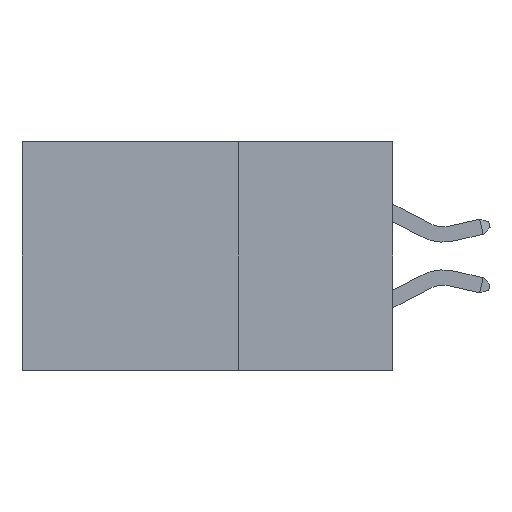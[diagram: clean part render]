
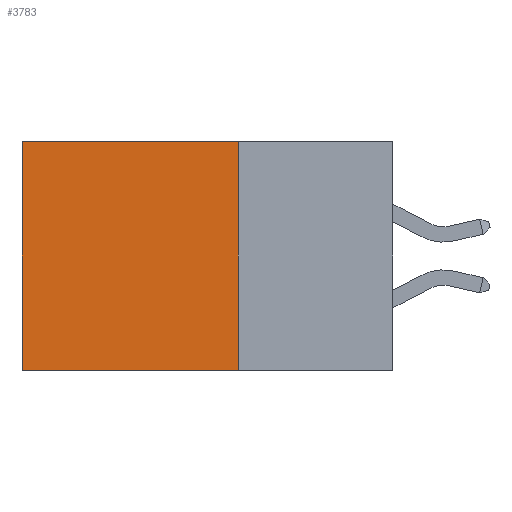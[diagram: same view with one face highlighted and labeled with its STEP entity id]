
A CAD part, left-side view. The second image highlights one B-rep face of the part: STEP entity #3783.
In plain terms, the highlighted planar face has unit normal (-1, 0, 0).
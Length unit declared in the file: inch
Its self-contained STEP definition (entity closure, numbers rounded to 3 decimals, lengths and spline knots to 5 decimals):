
#979 = ORIENTED_EDGE ( 'NONE', *, *, #10475, .F. ) ;
#1186 = DIRECTION ( 'NONE',  ( 0., 0., -1. ) ) ;
#1193 = VERTEX_POINT ( 'NONE', #20243 ) ;
#2127 = CARTESIAN_POINT ( 'NONE',  ( 0.2875, 0.6, -0.37 ) ) ;
#2405 = CARTESIAN_POINT ( 'NONE',  ( 0.2875, 0.25, -0.37 ) ) ;
#2890 = LINE ( 'NONE', #20522, #14597 ) ;
#3520 = VERTEX_POINT ( 'NONE', #20196 ) ;
#3783 = ADVANCED_FACE ( 'NONE', ( #15075 ), #10285, .F. ) ;
#3877 = VERTEX_POINT ( 'NONE', #4519 ) ;
#4420 = LINE ( 'NONE', #15878, #14667 ) ;
#4519 = CARTESIAN_POINT ( 'NONE',  ( 0.2875, 0.6, 0. ) ) ;
#4660 = DIRECTION ( 'NONE',  ( 0., 1., 0. ) ) ;
#7227 = DIRECTION ( 'NONE',  ( 1., 0., 0. ) ) ;
#8703 = DIRECTION ( 'NONE',  ( 0., 0., -1. ) ) ;
#9340 = ORIENTED_EDGE ( 'NONE', *, *, #15856, .T. ) ;
#9918 = VERTEX_POINT ( 'NONE', #2127 ) ;
#10285 = PLANE ( 'NONE',  #14788 ) ;
#10475 = EDGE_CURVE ( 'NONE', #1193, #9918, #16786, .T. ) ;
#11644 = EDGE_LOOP ( 'NONE', ( #9340, #979, #19516, #18137 ) ) ;
#11767 = VECTOR ( 'NONE', #12009, 39.37008 ) ;
#12009 = DIRECTION ( 'NONE',  ( 0., 1., 0. ) ) ;
#13523 = CARTESIAN_POINT ( 'NONE',  ( 0.2875, 0.6, 0. ) ) ;
#13703 = EDGE_CURVE ( 'NONE', #3520, #3877, #2890, .T. ) ;
#14597 = VECTOR ( 'NONE', #4660, 39.37008 ) ;
#14667 = VECTOR ( 'NONE', #1186, 39.37008 ) ;
#14788 = AXIS2_PLACEMENT_3D ( 'NONE', #16624, #7227, #8703 ) ;
#15075 = FACE_OUTER_BOUND ( 'NONE', #11644, .T. ) ;
#15856 = EDGE_CURVE ( 'NONE', #3877, #9918, #18198, .T. ) ;
#15878 = CARTESIAN_POINT ( 'NONE',  ( 0.2875, 0.25, 0. ) ) ;
#15972 = EDGE_CURVE ( 'NONE', #3520, #1193, #4420, .T. ) ;
#16624 = CARTESIAN_POINT ( 'NONE',  ( 0.2875, 0.25, 0. ) ) ;
#16786 = LINE ( 'NONE', #2405, #11767 ) ;
#18137 = ORIENTED_EDGE ( 'NONE', *, *, #13703, .T. ) ;
#18198 = LINE ( 'NONE', #13523, #18632 ) ;
#18632 = VECTOR ( 'NONE', #19864, 39.37008 ) ;
#19516 = ORIENTED_EDGE ( 'NONE', *, *, #15972, .F. ) ;
#19864 = DIRECTION ( 'NONE',  ( 0., 0., -1. ) ) ;
#20196 = CARTESIAN_POINT ( 'NONE',  ( 0.2875, 0.25, 0. ) ) ;
#20243 = CARTESIAN_POINT ( 'NONE',  ( 0.2875, 0.25, -0.37 ) ) ;
#20522 = CARTESIAN_POINT ( 'NONE',  ( 0.2875, 0.25, 0. ) ) ;
